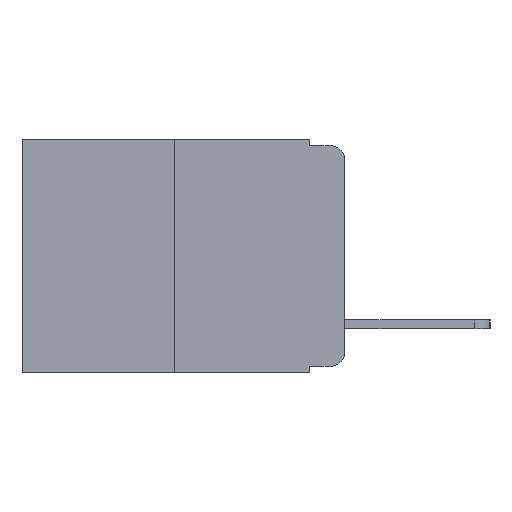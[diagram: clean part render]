
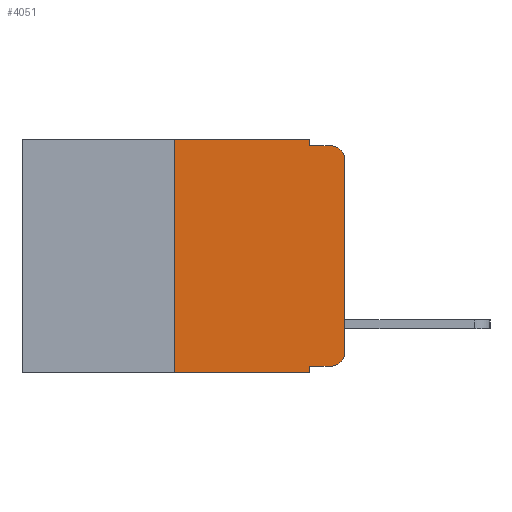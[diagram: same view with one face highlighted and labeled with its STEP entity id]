
A CAD part, left-side view. The second image highlights one B-rep face of the part: STEP entity #4051.
In plain terms, the highlighted planar face has unit normal (-1, 0, 0).
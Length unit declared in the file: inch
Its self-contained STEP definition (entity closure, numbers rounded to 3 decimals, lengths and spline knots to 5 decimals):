
#16 = VECTOR ( 'NONE', #4635, 39.37008 ) ;
#287 = CARTESIAN_POINT ( 'NONE',  ( 0., 0.051, -0.333 ) ) ;
#347 = FACE_OUTER_BOUND ( 'NONE', #5374, .T. ) ;
#352 = LINE ( 'NONE', #1456, #9725 ) ;
#570 = VERTEX_POINT ( 'NONE', #6716 ) ;
#600 = VERTEX_POINT ( 'NONE', #7960 ) ;
#838 = VERTEX_POINT ( 'NONE', #9163 ) ;
#975 = VERTEX_POINT ( 'NONE', #4177 ) ;
#1013 = ORIENTED_EDGE ( 'NONE', *, *, #11067, .T. ) ;
#1025 = CIRCLE ( 'NONE', #2950, 0.02 ) ;
#1108 = ORIENTED_EDGE ( 'NONE', *, *, #11119, .T. ) ;
#1456 = CARTESIAN_POINT ( 'NONE',  ( 0., 0.051, 0. ) ) ;
#1510 = ORIENTED_EDGE ( 'NONE', *, *, #11151, .F. ) ;
#1673 = ORIENTED_EDGE ( 'NONE', *, *, #11157, .F. ) ;
#1715 = ORIENTED_EDGE ( 'NONE', *, *, #10853, .F. ) ;
#1931 = ORIENTED_EDGE ( 'NONE', *, *, #11162, .F. ) ;
#1987 = ORIENTED_EDGE ( 'NONE', *, *, #10779, .T. ) ;
#2123 = LINE ( 'NONE', #8298, #8815 ) ;
#2362 = CARTESIAN_POINT ( 'NONE',  ( 0., 0.02, -0.03 ) ) ;
#2411 = VECTOR ( 'NONE', #9581, 39.37008 ) ;
#2457 = DIRECTION ( 'NONE',  ( 0., 0., -1. ) ) ;
#2559 = AXIS2_PLACEMENT_3D ( 'NONE', #2362, #8735, #3461 ) ;
#2812 = CARTESIAN_POINT ( 'NONE',  ( 0., 0.02, -0.01 ) ) ;
#2843 = VERTEX_POINT ( 'NONE', #2812 ) ;
#2950 = AXIS2_PLACEMENT_3D ( 'NONE', #9400, #4442, #10117 ) ;
#3087 = VECTOR ( 'NONE', #6374, 39.37008 ) ;
#3240 = ORIENTED_EDGE ( 'NONE', *, *, #11164, .F. ) ;
#3270 = ORIENTED_EDGE ( 'NONE', *, *, #11173, .T. ) ;
#3315 = CARTESIAN_POINT ( 'NONE',  ( 0., 0., 0. ) ) ;
#3461 = DIRECTION ( 'NONE',  ( 0., 0., -1. ) ) ;
#3572 = CARTESIAN_POINT ( 'NONE',  ( 0., 0.051, -0.333 ) ) ;
#4051 = ADVANCED_FACE ( 'NONE', ( #347 ), #4196, .F. ) ;
#4177 = CARTESIAN_POINT ( 'NONE',  ( 0., 0., -0.313 ) ) ;
#4182 = CARTESIAN_POINT ( 'NONE',  ( 0., 0.473, 0. ) ) ;
#4196 = PLANE ( 'NONE',  #8746 ) ;
#4261 = DIRECTION ( 'NONE',  ( 0., 0., -1. ) ) ;
#4273 = DIRECTION ( 'NONE',  ( 1., 0., 0. ) ) ;
#4429 = DIRECTION ( 'NONE',  ( 0., 0., 1. ) ) ;
#4442 = DIRECTION ( 'NONE',  ( -1., 0., 0. ) ) ;
#4635 = DIRECTION ( 'NONE',  ( 0., 0., 1. ) ) ;
#4684 = ORIENTED_EDGE ( 'NONE', *, *, #9315, .T. ) ;
#5208 = LINE ( 'NONE', #3572, #2411 ) ;
#5280 = VERTEX_POINT ( 'NONE', #9905 ) ;
#5362 = VERTEX_POINT ( 'NONE', #9236 ) ;
#5374 = EDGE_LOOP ( 'NONE', ( #1013, #1108, #1510, #1673, #1715, #1931, #1987, #3240, #3270, #4684 ) ) ;
#5813 = LINE ( 'NONE', #8765, #3087 ) ;
#6333 = VERTEX_POINT ( 'NONE', #7946 ) ;
#6374 = DIRECTION ( 'NONE',  ( 0., -1., 0. ) ) ;
#6403 = CARTESIAN_POINT ( 'NONE',  ( 0., 0.25, 0. ) ) ;
#6716 = CARTESIAN_POINT ( 'NONE',  ( 0., 0.25, 0. ) ) ;
#7081 = VECTOR ( 'NONE', #4429, 39.37008 ) ;
#7364 = LINE ( 'NONE', #10648, #11118 ) ;
#7469 = VECTOR ( 'NONE', #11025, 39.37008 ) ;
#7474 = DIRECTION ( 'NONE',  ( 0., -1., 0. ) ) ;
#7722 = LINE ( 'NONE', #10230, #7469 ) ;
#7946 = CARTESIAN_POINT ( 'NONE',  ( 0., 0.051, -0.343 ) ) ;
#7960 = CARTESIAN_POINT ( 'NONE',  ( 0., 0.051, -0.01 ) ) ;
#8210 = VERTEX_POINT ( 'NONE', #9966 ) ;
#8298 = CARTESIAN_POINT ( 'NONE',  ( 0., 0.473, -0.343 ) ) ;
#8450 = CIRCLE ( 'NONE', #2559, 0.02 ) ;
#8735 = DIRECTION ( 'NONE',  ( -1., 0., 0. ) ) ;
#8746 = AXIS2_PLACEMENT_3D ( 'NONE', #4182, #4273, #4261 ) ;
#8765 = CARTESIAN_POINT ( 'NONE',  ( 0., 0.051, -0.01 ) ) ;
#8815 = VECTOR ( 'NONE', #7474, 39.37008 ) ;
#9163 = CARTESIAN_POINT ( 'NONE',  ( 0., 0.25, -0.343 ) ) ;
#9236 = CARTESIAN_POINT ( 'NONE',  ( 0., 0.051, 0. ) ) ;
#9315 = EDGE_CURVE ( 'NONE', #8210, #975, #1025, .T. ) ;
#9400 = CARTESIAN_POINT ( 'NONE',  ( 0., 0.02, -0.313 ) ) ;
#9581 = DIRECTION ( 'NONE',  ( 0., -1., 0. ) ) ;
#9725 = VECTOR ( 'NONE', #2457, 39.37008 ) ;
#9905 = CARTESIAN_POINT ( 'NONE',  ( 0., 0., -0.03 ) ) ;
#9956 = LINE ( 'NONE', #6403, #16 ) ;
#9966 = CARTESIAN_POINT ( 'NONE',  ( 0., 0.02, -0.333 ) ) ;
#10117 = DIRECTION ( 'NONE',  ( 0., 0., -1. ) ) ;
#10230 = CARTESIAN_POINT ( 'NONE',  ( 0., 0.051, 0. ) ) ;
#10422 = VERTEX_POINT ( 'NONE', #287 ) ;
#10648 = CARTESIAN_POINT ( 'NONE',  ( 0., 0.473, 0. ) ) ;
#10779 = EDGE_CURVE ( 'NONE', #838, #6333, #2123, .T. ) ;
#10853 = EDGE_CURVE ( 'NONE', #570, #5362, #7364, .T. ) ;
#11025 = DIRECTION ( 'NONE',  ( 0., 0., -1. ) ) ;
#11067 = EDGE_CURVE ( 'NONE', #975, #5280, #11108, .T. ) ;
#11108 = LINE ( 'NONE', #3315, #7081 ) ;
#11118 = VECTOR ( 'NONE', #11371, 39.37008 ) ;
#11119 = EDGE_CURVE ( 'NONE', #5280, #2843, #8450, .T. ) ;
#11151 = EDGE_CURVE ( 'NONE', #600, #2843, #5813, .T. ) ;
#11157 = EDGE_CURVE ( 'NONE', #5362, #600, #352, .T. ) ;
#11162 = EDGE_CURVE ( 'NONE', #838, #570, #9956, .T. ) ;
#11164 = EDGE_CURVE ( 'NONE', #10422, #6333, #7722, .T. ) ;
#11173 = EDGE_CURVE ( 'NONE', #10422, #8210, #5208, .T. ) ;
#11371 = DIRECTION ( 'NONE',  ( 0., -1., 0. ) ) ;
